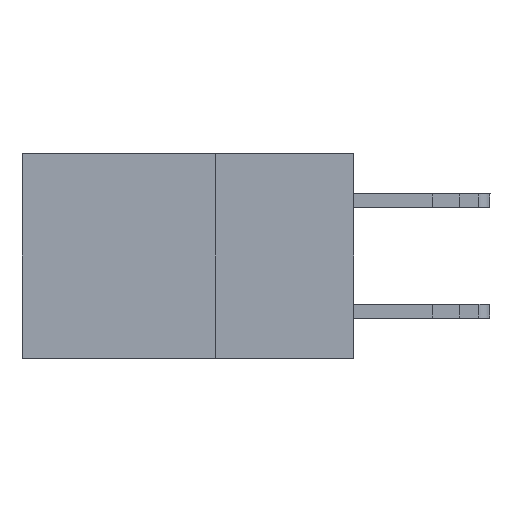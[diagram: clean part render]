
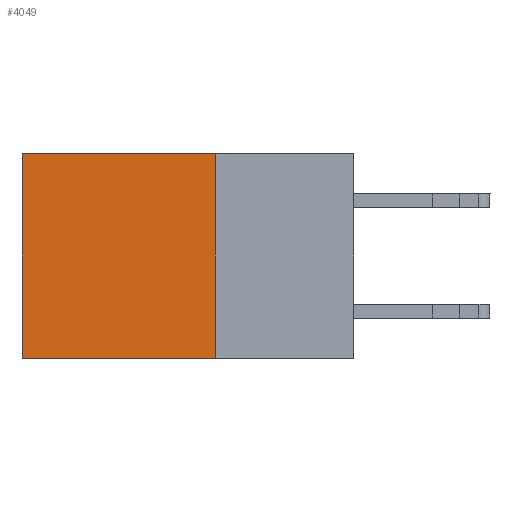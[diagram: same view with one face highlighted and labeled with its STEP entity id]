
A CAD part, left-side view. The second image highlights one B-rep face of the part: STEP entity #4049.
In plain terms, the highlighted planar face has unit normal (-1, 0, 0).
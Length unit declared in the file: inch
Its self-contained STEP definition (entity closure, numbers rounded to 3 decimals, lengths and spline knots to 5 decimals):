
#900 = CARTESIAN_POINT ( 'NONE',  ( 0.2875, 0.25, -0.37 ) ) ;
#1601 = ORIENTED_EDGE ( 'NONE', *, *, #21763, .T. ) ;
#2637 = VECTOR ( 'NONE', #5221, 39.37008 ) ;
#3668 = CARTESIAN_POINT ( 'NONE',  ( 0.2875, 0.6, -0.37 ) ) ;
#4049 = ADVANCED_FACE ( 'NONE', ( #15913 ), #13947, .F. ) ;
#4591 = DIRECTION ( 'NONE',  ( 0., 0., -1. ) ) ;
#5221 = DIRECTION ( 'NONE',  ( 0., 0., -1. ) ) ;
#7127 = ORIENTED_EDGE ( 'NONE', *, *, #8462, .T. ) ;
#7544 = DIRECTION ( 'NONE',  ( 0., 1., 0. ) ) ;
#8228 = LINE ( 'NONE', #8925, #20145 ) ;
#8462 = EDGE_CURVE ( 'NONE', #11589, #14983, #11673, .T. ) ;
#8925 = CARTESIAN_POINT ( 'NONE',  ( 0.2875, 0.25, 0. ) ) ;
#9227 = LINE ( 'NONE', #900, #17729 ) ;
#9970 = VECTOR ( 'NONE', #25611, 39.37008 ) ;
#10894 = EDGE_CURVE ( 'NONE', #19419, #23709, #9227, .T. ) ;
#11589 = VERTEX_POINT ( 'NONE', #16721 ) ;
#11673 = LINE ( 'NONE', #14491, #9970 ) ;
#12591 = AXIS2_PLACEMENT_3D ( 'NONE', #20705, #18224, #14152 ) ;
#12945 = CARTESIAN_POINT ( 'NONE',  ( 0.2875, 0.25, -0.37 ) ) ;
#13947 = PLANE ( 'NONE',  #12591 ) ;
#14152 = DIRECTION ( 'NONE',  ( 0., 0., -1. ) ) ;
#14491 = CARTESIAN_POINT ( 'NONE',  ( 0.2875, 0.25, 0. ) ) ;
#14983 = VERTEX_POINT ( 'NONE', #24830 ) ;
#15468 = ORIENTED_EDGE ( 'NONE', *, *, #10894, .F. ) ;
#15913 = FACE_OUTER_BOUND ( 'NONE', #18767, .T. ) ;
#16721 = CARTESIAN_POINT ( 'NONE',  ( 0.2875, 0.25, 0. ) ) ;
#17729 = VECTOR ( 'NONE', #7544, 39.37008 ) ;
#18224 = DIRECTION ( 'NONE',  ( 1., 0., 0. ) ) ;
#18767 = EDGE_LOOP ( 'NONE', ( #1601, #15468, #18931, #7127 ) ) ;
#18931 = ORIENTED_EDGE ( 'NONE', *, *, #26627, .F. ) ;
#19077 = LINE ( 'NONE', #22901, #2637 ) ;
#19419 = VERTEX_POINT ( 'NONE', #12945 ) ;
#20145 = VECTOR ( 'NONE', #4591, 39.37008 ) ;
#20705 = CARTESIAN_POINT ( 'NONE',  ( 0.2875, 0.25, 0. ) ) ;
#21763 = EDGE_CURVE ( 'NONE', #14983, #23709, #19077, .T. ) ;
#22901 = CARTESIAN_POINT ( 'NONE',  ( 0.2875, 0.6, 0. ) ) ;
#23709 = VERTEX_POINT ( 'NONE', #3668 ) ;
#24830 = CARTESIAN_POINT ( 'NONE',  ( 0.2875, 0.6, 0. ) ) ;
#25611 = DIRECTION ( 'NONE',  ( 0., 1., 0. ) ) ;
#26627 = EDGE_CURVE ( 'NONE', #11589, #19419, #8228, .T. ) ;
